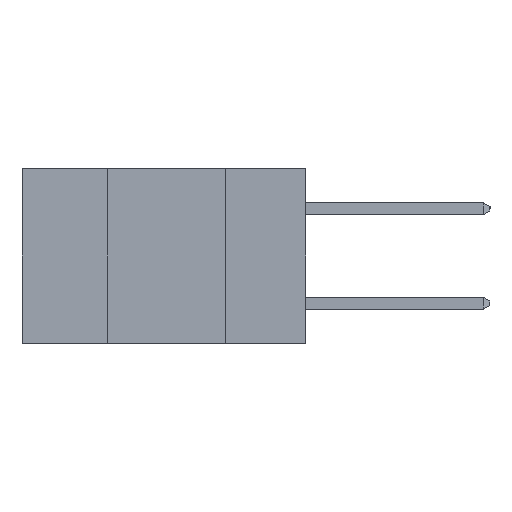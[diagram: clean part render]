
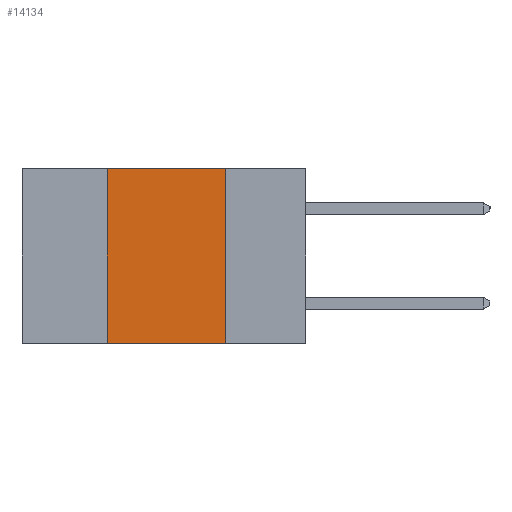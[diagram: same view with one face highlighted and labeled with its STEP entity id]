
A CAD part, left-side view. The second image highlights one B-rep face of the part: STEP entity #14134.
In plain terms, the highlighted planar face has unit normal (-1, 0, 0).
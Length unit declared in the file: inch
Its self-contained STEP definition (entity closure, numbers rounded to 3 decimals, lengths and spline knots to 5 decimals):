
#900 = VERTEX_POINT ( 'NONE', #21738 ) ;
#1209 = DIRECTION ( 'NONE',  ( 1., 0., 0. ) ) ;
#1449 = ORIENTED_EDGE ( 'NONE', *, *, #15498, .T. ) ;
#1968 = AXIS2_PLACEMENT_3D ( 'NONE', #15480, #1209, #23744 ) ;
#2368 = VECTOR ( 'NONE', #19906, 39.37008 ) ;
#2925 = FACE_OUTER_BOUND ( 'NONE', #26147, .T. ) ;
#3919 = VECTOR ( 'NONE', #19144, 39.37008 ) ;
#5617 = CARTESIAN_POINT ( 'NONE',  ( 0., 0.17, -0.37 ) ) ;
#6137 = CARTESIAN_POINT ( 'NONE',  ( 0., 0.42, -0.37 ) ) ;
#7189 = LINE ( 'NONE', #15316, #19872 ) ;
#7714 = VERTEX_POINT ( 'NONE', #15259 ) ;
#8186 = CARTESIAN_POINT ( 'NONE',  ( 0., 0.17, -0.37 ) ) ;
#8899 = LINE ( 'NONE', #17288, #3919 ) ;
#10204 = EDGE_CURVE ( 'NONE', #900, #7714, #8899, .T. ) ;
#11649 = ORIENTED_EDGE ( 'NONE', *, *, #12520, .F. ) ;
#12520 = EDGE_CURVE ( 'NONE', #7714, #23128, #20169, .T. ) ;
#14134 = ADVANCED_FACE ( 'NONE', ( #2925 ), #23347, .F. ) ;
#14400 = VERTEX_POINT ( 'NONE', #6137 ) ;
#14764 = VECTOR ( 'NONE', #24559, 39.37008 ) ;
#14843 = EDGE_CURVE ( 'NONE', #14400, #900, #7189, .T. ) ;
#15259 = CARTESIAN_POINT ( 'NONE',  ( 0., 0.17, 0. ) ) ;
#15316 = CARTESIAN_POINT ( 'NONE',  ( 0., 0.42, -0.37 ) ) ;
#15480 = CARTESIAN_POINT ( 'NONE',  ( 0., 0.6, 0. ) ) ;
#15498 = EDGE_CURVE ( 'NONE', #14400, #23128, #16423, .T. ) ;
#16423 = LINE ( 'NONE', #18177, #14764 ) ;
#17288 = CARTESIAN_POINT ( 'NONE',  ( 0., 0.6, 0. ) ) ;
#18177 = CARTESIAN_POINT ( 'NONE',  ( 0., 0.6, -0.37 ) ) ;
#19144 = DIRECTION ( 'NONE',  ( 0., -1., 0. ) ) ;
#19872 = VECTOR ( 'NONE', #23442, 39.37008 ) ;
#19906 = DIRECTION ( 'NONE',  ( 0., 0., -1. ) ) ;
#20169 = LINE ( 'NONE', #8186, #2368 ) ;
#21105 = ORIENTED_EDGE ( 'NONE', *, *, #10204, .F. ) ;
#21738 = CARTESIAN_POINT ( 'NONE',  ( 0., 0.42, 0. ) ) ;
#23128 = VERTEX_POINT ( 'NONE', #5617 ) ;
#23347 = PLANE ( 'NONE',  #1968 ) ;
#23421 = ORIENTED_EDGE ( 'NONE', *, *, #14843, .F. ) ;
#23442 = DIRECTION ( 'NONE',  ( 0., 0., 1. ) ) ;
#23744 = DIRECTION ( 'NONE',  ( 0., 0., -1. ) ) ;
#24559 = DIRECTION ( 'NONE',  ( 0., -1., 0. ) ) ;
#26147 = EDGE_LOOP ( 'NONE', ( #11649, #21105, #23421, #1449 ) ) ;
